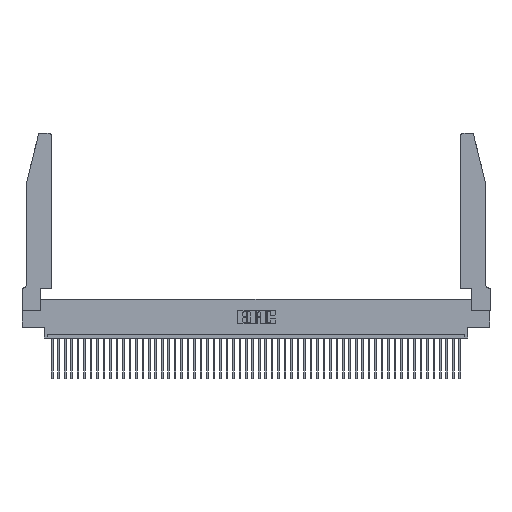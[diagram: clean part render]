
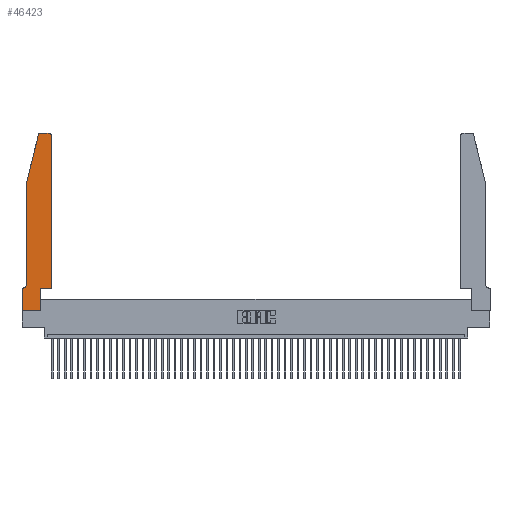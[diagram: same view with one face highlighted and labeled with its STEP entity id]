
A CAD part, top view. The second image highlights one B-rep face of the part: STEP entity #46423.
In plain terms, the highlighted planar face has unit normal (0, 0, 1).
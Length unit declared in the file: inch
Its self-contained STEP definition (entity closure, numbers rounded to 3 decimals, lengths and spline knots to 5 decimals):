
#1289 = CARTESIAN_POINT ( 'NONE',  ( 0.2865, 0.35, 0.37 ) ) ;
#1353 = CARTESIAN_POINT ( 'NONE',  ( 0.4505, 0.35, 0.37 ) ) ;
#2206 = DIRECTION ( 'NONE',  ( -1., 0., 0. ) ) ;
#4017 = ORIENTED_EDGE ( 'NONE', *, *, #28684, .T. ) ;
#4129 = VERTEX_POINT ( 'NONE', #18862 ) ;
#5409 = AXIS2_PLACEMENT_3D ( 'NONE', #40936, #33195, #18246 ) ;
#5450 = CIRCLE ( 'NONE', #7165, 0.07 ) ;
#6467 = VECTOR ( 'NONE', #39926, 39.37008 ) ;
#6953 = ORIENTED_EDGE ( 'NONE', *, *, #29672, .T. ) ;
#7165 = AXIS2_PLACEMENT_3D ( 'NONE', #39916, #47033, #16729 ) ;
#7299 = CARTESIAN_POINT ( 'NONE',  ( 0.2865, 0., 0.37 ) ) ;
#7666 = VECTOR ( 'NONE', #20204, 39.37008 ) ;
#8655 = LINE ( 'NONE', #29528, #30469 ) ;
#8720 = VERTEX_POINT ( 'NONE', #12041 ) ;
#9086 = DIRECTION ( 'NONE',  ( 0., 0., 1. ) ) ;
#9164 = EDGE_CURVE ( 'NONE', #14253, #45413, #50092, .T. ) ;
#9444 = LINE ( 'NONE', #27864, #39129 ) ;
#9534 = VECTOR ( 'NONE', #15199, 39.37008 ) ;
#9554 = LINE ( 'NONE', #42592, #30150 ) ;
#10066 = ORIENTED_EDGE ( 'NONE', *, *, #29024, .T. ) ;
#10479 = FACE_OUTER_BOUND ( 'NONE', #47259, .T. ) ;
#11745 = CARTESIAN_POINT ( 'NONE',  ( 0.2865, 0.35, 0.37 ) ) ;
#12041 = CARTESIAN_POINT ( 'NONE',  ( 0., 0., 0.37 ) ) ;
#12201 = VERTEX_POINT ( 'NONE', #32922 ) ;
#12316 = VERTEX_POINT ( 'NONE', #7299 ) ;
#13415 = CIRCLE ( 'NONE', #41423, 0.03 ) ;
#14253 = VERTEX_POINT ( 'NONE', #42081 ) ;
#14640 = ORIENTED_EDGE ( 'NONE', *, *, #17386, .T. ) ;
#14728 = CARTESIAN_POINT ( 'NONE',  ( 0.4505, 0.35, 0.37 ) ) ;
#15199 = DIRECTION ( 'NONE',  ( -1., 0., 0. ) ) ;
#16608 = VERTEX_POINT ( 'NONE', #34812 ) ;
#16698 = DIRECTION ( 'NONE',  ( 1., 0., 0. ) ) ;
#16729 = DIRECTION ( 'NONE',  ( -1., 0., 0. ) ) ;
#17336 = DIRECTION ( 'NONE',  ( -0.239, -0.971, 0. ) ) ;
#17386 = EDGE_CURVE ( 'NONE', #8720, #12316, #8655, .T. ) ;
#17998 = CARTESIAN_POINT ( 'NONE',  ( 0.4505, 0.35, 0.37 ) ) ;
#18113 = EDGE_CURVE ( 'NONE', #18959, #4129, #13415, .T. ) ;
#18246 = DIRECTION ( 'NONE',  ( 1., 0., 0. ) ) ;
#18591 = DIRECTION ( 'NONE',  ( 0., 1., 0. ) ) ;
#18637 = CARTESIAN_POINT ( 'NONE',  ( 0., 0.35, 0.37 ) ) ;
#18862 = CARTESIAN_POINT ( 'NONE',  ( 0.25487, 2.72718, 0.37 ) ) ;
#18959 = VERTEX_POINT ( 'NONE', #25483 ) ;
#19373 = CIRCLE ( 'NONE', #5409, 0.03 ) ;
#19893 = VERTEX_POINT ( 'NONE', #35945 ) ;
#20109 = ORIENTED_EDGE ( 'NONE', *, *, #40756, .T. ) ;
#20182 = EDGE_CURVE ( 'NONE', #19893, #18959, #41624, .T. ) ;
#20204 = DIRECTION ( 'NONE',  ( 0., 1., 0. ) ) ;
#20722 = ORIENTED_EDGE ( 'NONE', *, *, #9164, .T. ) ;
#20772 = DIRECTION ( 'NONE',  ( 1., 0., 0. ) ) ;
#22530 = LINE ( 'NONE', #44863, #41876 ) ;
#23475 = VERTEX_POINT ( 'NONE', #17998 ) ;
#24128 = ORIENTED_EDGE ( 'NONE', *, *, #47106, .T. ) ;
#24497 = DIRECTION ( 'NONE',  ( 0., 0., 1. ) ) ;
#24779 = ORIENTED_EDGE ( 'NONE', *, *, #20182, .T. ) ;
#25302 = VECTOR ( 'NONE', #2206, 39.37008 ) ;
#25483 = CARTESIAN_POINT ( 'NONE',  ( 0.284, 2.75, 0.37 ) ) ;
#26662 = EDGE_CURVE ( 'NONE', #48364, #23475, #37385, .T. ) ;
#27196 = DIRECTION ( 'NONE',  ( 0., -1., 0. ) ) ;
#27307 = EDGE_CURVE ( 'NONE', #45413, #8720, #9444, .T. ) ;
#27864 = CARTESIAN_POINT ( 'NONE',  ( 0., 0., 0.37 ) ) ;
#28684 = EDGE_CURVE ( 'NONE', #29207, #19893, #19373, .T. ) ;
#28882 = ORIENTED_EDGE ( 'NONE', *, *, #34179, .T. ) ;
#29024 = EDGE_CURVE ( 'NONE', #16608, #12201, #9554, .T. ) ;
#29207 = VERTEX_POINT ( 'NONE', #48457 ) ;
#29528 = CARTESIAN_POINT ( 'NONE',  ( 0., 0., 0.37 ) ) ;
#29672 = EDGE_CURVE ( 'NONE', #12316, #48364, #43978, .T. ) ;
#30150 = VECTOR ( 'NONE', #27196, 39.37008 ) ;
#30469 = VECTOR ( 'NONE', #49465, 39.37008 ) ;
#32922 = CARTESIAN_POINT ( 'NONE',  ( 0.0755, 0.42, 0.37 ) ) ;
#33195 = DIRECTION ( 'NONE',  ( 0., 0., 1. ) ) ;
#34179 = EDGE_CURVE ( 'NONE', #12201, #14253, #5450, .T. ) ;
#34812 = CARTESIAN_POINT ( 'NONE',  ( 0.0755, 2., 0.37 ) ) ;
#35945 = CARTESIAN_POINT ( 'NONE',  ( 0.4205, 2.75, 0.37 ) ) ;
#36036 = PLANE ( 'NONE',  #36053 ) ;
#36053 = AXIS2_PLACEMENT_3D ( 'NONE', #39896, #9086, #16698 ) ;
#36179 = CARTESIAN_POINT ( 'NONE',  ( 0.284, 2.72, 0.37 ) ) ;
#37385 = LINE ( 'NONE', #1353, #6467 ) ;
#38405 = CARTESIAN_POINT ( 'NONE',  ( 0.2605, 2.75, 0.37 ) ) ;
#39129 = VECTOR ( 'NONE', #46986, 39.37008 ) ;
#39896 = CARTESIAN_POINT ( 'NONE',  ( 0., 0.35, 0.37 ) ) ;
#39916 = CARTESIAN_POINT ( 'NONE',  ( 0.0055, 0.42, 0.37 ) ) ;
#39926 = DIRECTION ( 'NONE',  ( 1., 0., 0. ) ) ;
#40756 = EDGE_CURVE ( 'NONE', #23475, #29207, #49951, .T. ) ;
#40936 = CARTESIAN_POINT ( 'NONE',  ( 0.4205, 2.72, 0.37 ) ) ;
#41323 = ORIENTED_EDGE ( 'NONE', *, *, #26662, .T. ) ;
#41423 = AXIS2_PLACEMENT_3D ( 'NONE', #36179, #24497, #20772 ) ;
#41624 = LINE ( 'NONE', #38405, #9534 ) ;
#41876 = VECTOR ( 'NONE', #17336, 39.37008 ) ;
#42081 = CARTESIAN_POINT ( 'NONE',  ( 0.0055, 0.35, 0.37 ) ) ;
#42102 = VECTOR ( 'NONE', #18591, 39.37008 ) ;
#42592 = CARTESIAN_POINT ( 'NONE',  ( 0.0755, 2., 0.37 ) ) ;
#43978 = LINE ( 'NONE', #11745, #7666 ) ;
#44863 = CARTESIAN_POINT ( 'NONE',  ( 0.0755, 2., 0.37 ) ) ;
#44956 = ORIENTED_EDGE ( 'NONE', *, *, #27307, .T. ) ;
#45413 = VERTEX_POINT ( 'NONE', #18637 ) ;
#46291 = ORIENTED_EDGE ( 'NONE', *, *, #18113, .T. ) ;
#46423 = ADVANCED_FACE ( 'NONE', ( #10479 ), #36036, .T. ) ;
#46986 = DIRECTION ( 'NONE',  ( 0., -1., 0. ) ) ;
#47033 = DIRECTION ( 'NONE',  ( 0., 0., -1. ) ) ;
#47106 = EDGE_CURVE ( 'NONE', #4129, #16608, #22530, .T. ) ;
#47259 = EDGE_LOOP ( 'NONE', ( #24779, #46291, #24128, #10066, #28882, #20722, #44956, #14640, #6953, #41323, #20109, #4017 ) ) ;
#48364 = VERTEX_POINT ( 'NONE', #1289 ) ;
#48457 = CARTESIAN_POINT ( 'NONE',  ( 0.4505, 2.72, 0.37 ) ) ;
#48516 = CARTESIAN_POINT ( 'NONE',  ( 0.0755, 0.35, 0.37 ) ) ;
#49465 = DIRECTION ( 'NONE',  ( 1., 0., 0. ) ) ;
#49951 = LINE ( 'NONE', #14728, #42102 ) ;
#50092 = LINE ( 'NONE', #48516, #25302 ) ;
